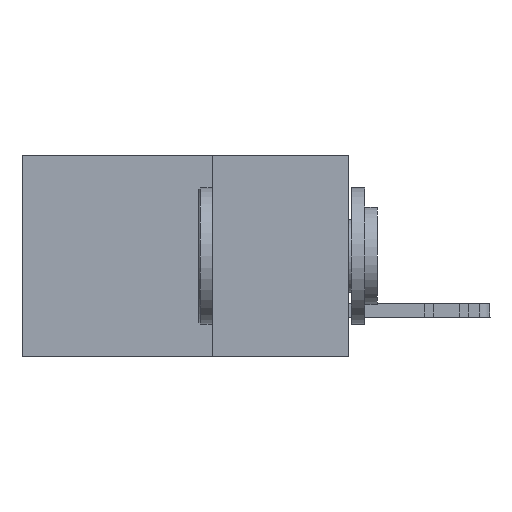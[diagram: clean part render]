
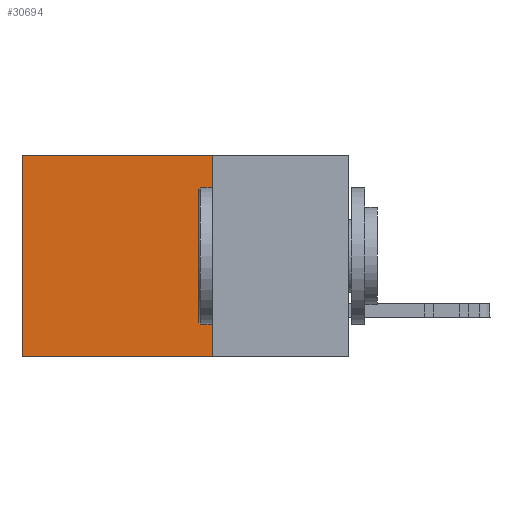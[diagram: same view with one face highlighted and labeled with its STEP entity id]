
A CAD part, left-side view. The second image highlights one B-rep face of the part: STEP entity #30694.
In plain terms, the highlighted planar face has unit normal (-1, 0, 0).
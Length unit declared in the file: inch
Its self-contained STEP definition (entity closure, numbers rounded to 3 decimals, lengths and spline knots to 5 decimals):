
#1824 = FACE_OUTER_BOUND ( 'NONE', #11946, .T. ) ;
#2459 = PLANE ( 'NONE',  #10544 ) ;
#2988 = EDGE_CURVE ( 'NONE', #14627, #16942, #9467, .T. ) ;
#3990 = ORIENTED_EDGE ( 'NONE', *, *, #2988, .T. ) ;
#4926 = EDGE_CURVE ( 'NONE', #16942, #11703, #17743, .T. ) ;
#5767 = VERTEX_POINT ( 'NONE', #18145 ) ;
#6806 = DIRECTION ( 'NONE',  ( 0., 0., -1. ) ) ;
#6857 = ORIENTED_EDGE ( 'NONE', *, *, #4926, .T. ) ;
#7223 = CARTESIAN_POINT ( 'NONE',  ( 0.298, 0.25, 0. ) ) ;
#8626 = DIRECTION ( 'NONE',  ( 0., 1., 0. ) ) ;
#8935 = CARTESIAN_POINT ( 'NONE',  ( 0.298, 0.25, 0. ) ) ;
#9467 = LINE ( 'NONE', #7223, #13199 ) ;
#9677 = CARTESIAN_POINT ( 'NONE',  ( 0.298, 0.25, 0. ) ) ;
#10544 = AXIS2_PLACEMENT_3D ( 'NONE', #9677, #24045, #6806 ) ;
#10651 = LINE ( 'NONE', #15971, #29360 ) ;
#10808 = DIRECTION ( 'NONE',  ( 0., 0., -1. ) ) ;
#10932 = EDGE_CURVE ( 'NONE', #14627, #5767, #10651, .T. ) ;
#11703 = VERTEX_POINT ( 'NONE', #24078 ) ;
#11946 = EDGE_LOOP ( 'NONE', ( #6857, #22471, #18798, #3990 ) ) ;
#12734 = CARTESIAN_POINT ( 'NONE',  ( 0.298, 0.6, 0. ) ) ;
#13053 = VECTOR ( 'NONE', #8626, 39.37008 ) ;
#13199 = VECTOR ( 'NONE', #26228, 39.37008 ) ;
#14627 = VERTEX_POINT ( 'NONE', #8935 ) ;
#15907 = CARTESIAN_POINT ( 'NONE',  ( 0.298, 0.25, -0.37 ) ) ;
#15971 = CARTESIAN_POINT ( 'NONE',  ( 0.298, 0.25, 0. ) ) ;
#16942 = VERTEX_POINT ( 'NONE', #12734 ) ;
#17147 = CARTESIAN_POINT ( 'NONE',  ( 0.298, 0.6, 0. ) ) ;
#17743 = LINE ( 'NONE', #17147, #18419 ) ;
#18145 = CARTESIAN_POINT ( 'NONE',  ( 0.298, 0.25, -0.37 ) ) ;
#18419 = VECTOR ( 'NONE', #31300, 39.37008 ) ;
#18631 = LINE ( 'NONE', #15907, #13053 ) ;
#18798 = ORIENTED_EDGE ( 'NONE', *, *, #10932, .F. ) ;
#21767 = EDGE_CURVE ( 'NONE', #5767, #11703, #18631, .T. ) ;
#22471 = ORIENTED_EDGE ( 'NONE', *, *, #21767, .F. ) ;
#24045 = DIRECTION ( 'NONE',  ( 1., 0., 0. ) ) ;
#24078 = CARTESIAN_POINT ( 'NONE',  ( 0.298, 0.6, -0.37 ) ) ;
#26228 = DIRECTION ( 'NONE',  ( 0., 1., 0. ) ) ;
#29360 = VECTOR ( 'NONE', #10808, 39.37008 ) ;
#30694 = ADVANCED_FACE ( 'NONE', ( #1824 ), #2459, .F. ) ;
#31300 = DIRECTION ( 'NONE',  ( 0., 0., -1. ) ) ;
